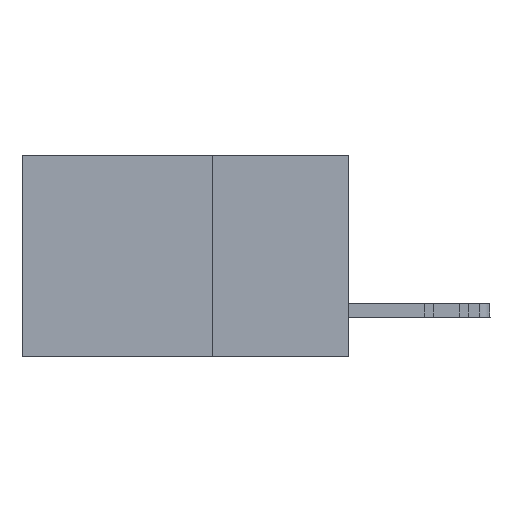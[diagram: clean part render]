
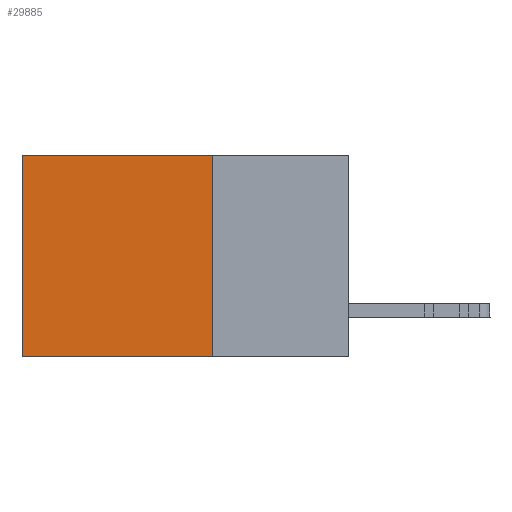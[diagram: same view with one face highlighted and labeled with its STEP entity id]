
A CAD part, left-side view. The second image highlights one B-rep face of the part: STEP entity #29885.
In plain terms, the highlighted planar face has unit normal (-1, 0, 0).
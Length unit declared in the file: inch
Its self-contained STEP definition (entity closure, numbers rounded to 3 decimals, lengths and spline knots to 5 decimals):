
#657 = LINE ( 'NONE', #20115, #2661 ) ;
#2384 = LINE ( 'NONE', #14899, #20568 ) ;
#2661 = VECTOR ( 'NONE', #18001, 39.37008 ) ;
#2860 = DIRECTION ( 'NONE',  ( 0., 1., 0. ) ) ;
#4357 = DIRECTION ( 'NONE',  ( 0., 0., -1. ) ) ;
#4848 = LINE ( 'NONE', #24475, #31345 ) ;
#6797 = EDGE_CURVE ( 'NONE', #28963, #25693, #2384, .T. ) ;
#7116 = EDGE_CURVE ( 'NONE', #28963, #14585, #25299, .T. ) ;
#7947 = ORIENTED_EDGE ( 'NONE', *, *, #7116, .F. ) ;
#9024 = FACE_OUTER_BOUND ( 'NONE', #10893, .T. ) ;
#9485 = PLANE ( 'NONE',  #30311 ) ;
#10252 = VECTOR ( 'NONE', #18213, 39.37008 ) ;
#10893 = EDGE_LOOP ( 'NONE', ( #11865, #27472, #7947, #28810 ) ) ;
#10936 = CARTESIAN_POINT ( 'NONE',  ( 0.298, 0.6, -0.37 ) ) ;
#11384 = CARTESIAN_POINT ( 'NONE',  ( 0.298, 0.25, 0. ) ) ;
#11865 = ORIENTED_EDGE ( 'NONE', *, *, #28587, .T. ) ;
#12885 = VERTEX_POINT ( 'NONE', #10936 ) ;
#14585 = VERTEX_POINT ( 'NONE', #15222 ) ;
#14899 = CARTESIAN_POINT ( 'NONE',  ( 0.298, 0.25, 0. ) ) ;
#15222 = CARTESIAN_POINT ( 'NONE',  ( 0.298, 0.25, -0.37 ) ) ;
#15790 = CARTESIAN_POINT ( 'NONE',  ( 0.298, 0.6, 0. ) ) ;
#18001 = DIRECTION ( 'NONE',  ( 0., 1., 0. ) ) ;
#18003 = EDGE_CURVE ( 'NONE', #14585, #12885, #657, .T. ) ;
#18213 = DIRECTION ( 'NONE',  ( 0., 0., -1. ) ) ;
#18670 = CARTESIAN_POINT ( 'NONE',  ( 0.298, 0.25, 0. ) ) ;
#20115 = CARTESIAN_POINT ( 'NONE',  ( 0.298, 0.25, -0.37 ) ) ;
#20568 = VECTOR ( 'NONE', #2860, 39.37008 ) ;
#21451 = DIRECTION ( 'NONE',  ( 0., 0., -1. ) ) ;
#24475 = CARTESIAN_POINT ( 'NONE',  ( 0.298, 0.6, 0. ) ) ;
#25299 = LINE ( 'NONE', #25780, #10252 ) ;
#25693 = VERTEX_POINT ( 'NONE', #15790 ) ;
#25780 = CARTESIAN_POINT ( 'NONE',  ( 0.298, 0.25, 0. ) ) ;
#27472 = ORIENTED_EDGE ( 'NONE', *, *, #18003, .F. ) ;
#28587 = EDGE_CURVE ( 'NONE', #25693, #12885, #4848, .T. ) ;
#28640 = DIRECTION ( 'NONE',  ( 1., 0., 0. ) ) ;
#28810 = ORIENTED_EDGE ( 'NONE', *, *, #6797, .T. ) ;
#28963 = VERTEX_POINT ( 'NONE', #11384 ) ;
#29885 = ADVANCED_FACE ( 'NONE', ( #9024 ), #9485, .F. ) ;
#30311 = AXIS2_PLACEMENT_3D ( 'NONE', #18670, #28640, #4357 ) ;
#31345 = VECTOR ( 'NONE', #21451, 39.37008 ) ;
